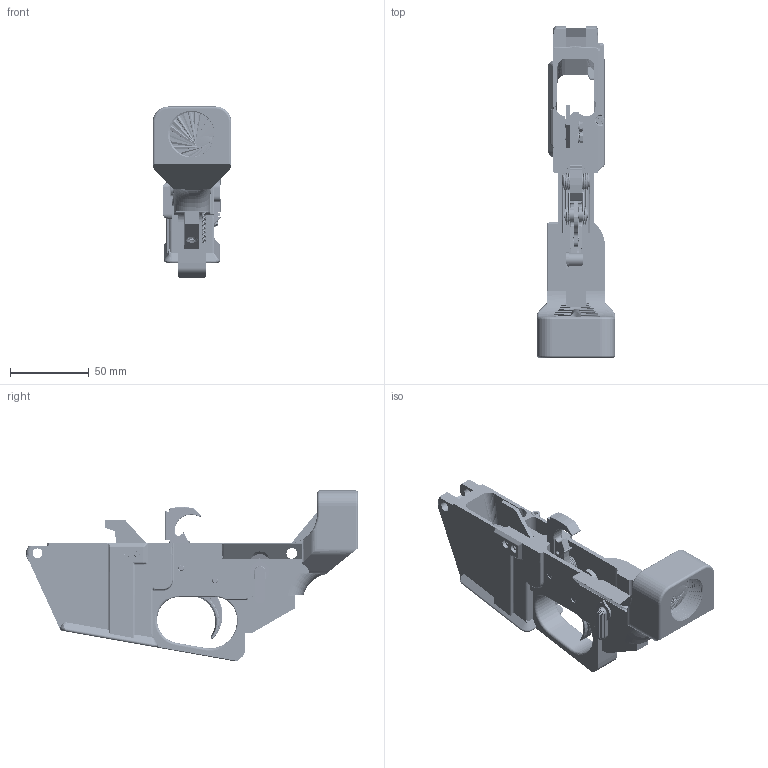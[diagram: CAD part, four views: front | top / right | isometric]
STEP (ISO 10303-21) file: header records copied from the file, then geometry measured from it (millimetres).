
FILE_DESCRIPTION(/* description */ (''),/* implementation_level */ '2;1');
FILE_NAME(/* name */ '(Unsaved).step',/* time_stamp */ '2019-07-03T20:59:34-04:00',/* author */ (''),/* organization */ (''),/* preprocessor_version */ 'ST-DEVELOPER v18',/* originating_system */ 'Autodesk Translation Framework v8.2.0.1029',/* authorisation */ '');
FILE_SCHEMA (('AUTOMOTIVE_DESIGN { 1 0 10303 214 3 1 1 }'));
Products named in the file (28): (Unsaved); Component1; trigger (1); trigger; Fire Control Group; Hammer Assembly; Hammer; Hammer Pin Retaining Spring J-Pin; Hammer Spring; Hammer Pin; Trigger Assembly; Trigger_1; Trigger Spring; Trigger Disconnector Spring; Trigger Disconnector; Trigger Pin; Fire Selector Assembly; Fire Selector Detent; Fire Selector; Fire Selector Spring; mag release; AR9 MagRelease v1; 91290A136; AR9 Ejector v1; ar9 (3); 91290A572; 90591A250; 90965A130
Assembly tree (31 placements, depth 7):
  (Unsaved)
    Component1
      trigger (1)
        trigger
          Fire Control Group
            Hammer Assembly
              Hammer
              Hammer Pin Retaining Spring J-Pin
              Hammer Spring
              Hammer Pin
            Trigger Assembly
              Trigger_1
              Trigger Spring
              Trigger Disconnector Spring
              Trigger Disconnector
              Trigger Pin
            Fire Selector Assembly
              Fire Selector Detent
              Fire Selector
              Fire Selector Spring
        mag release
          AR9 MagRelease v1
        91290A136
        90591A250  x2
    AR9 Ejector v1
    91290A572  x2
    90965A130  x2
    ar9 (3)
    90591A250
Bounding box: 50.01 x 211.38 x 108.92 mm (x, y, z)
Volume: 193311.5 mm3; surface area: 77865.2 mm2
Topology: 23 solids, 23 shells, 1735 faces, 4801 edges, 3080 vertices
Faces by surface type: cylinder 754, plane 509, bspline 203, torus 144, cone 103, sphere 22
Full cylindrical faces by diameter (mm): 0.889 x5, 1.143 x7, 1.372 x1, 1.934 x1, 2.35 x100, 2.362 x1, 2.438 x1, 2.464 x1, 2.529 x21, 2.54 x1, 3 x112, 3.023 x1, 3.048 x1, 3.086 x4, 3.175 x1, 3.2 x3, 3.556 x1, 3.912 x8, 3.962 x8, 4.216 x1, 5.172 x21, 5.334 x2, 5.5 x3, 6.35 x21, 6.375 x2, 6.477 x1, 6.858 x1, 7 x2, 7.044 x2, 7.861 x1
Entity records: 133056 total; most frequent: CARTESIAN_POINT 93875, ORIENTED_EDGE 8690, DIRECTION 7398, EDGE_CURVE 4345, AXIS2_PLACEMENT_3D 2848, VERTEX_POINT 2814, LINE 1702, VECTOR 1702
